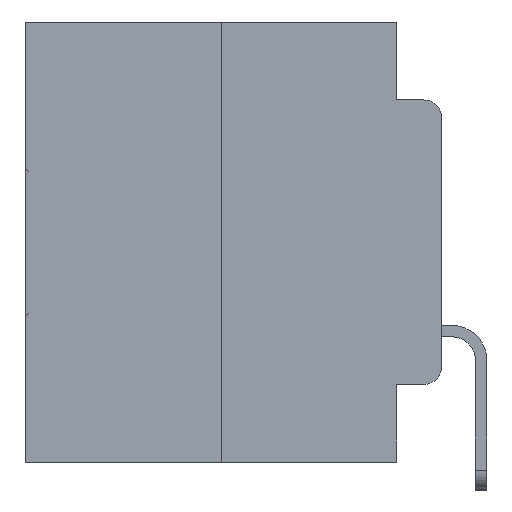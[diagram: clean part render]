
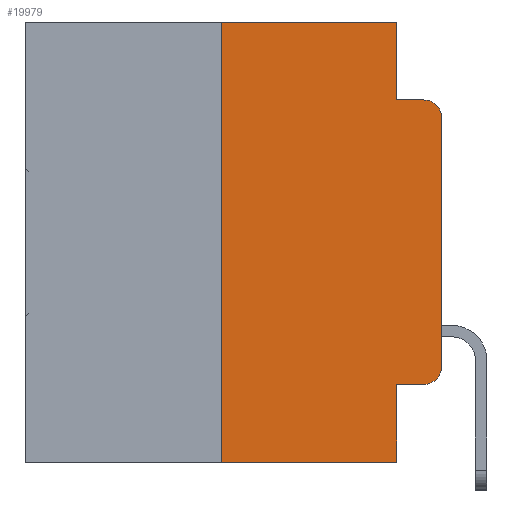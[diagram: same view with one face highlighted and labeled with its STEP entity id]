
A CAD part, left-side view. The second image highlights one B-rep face of the part: STEP entity #19979.
In plain terms, the highlighted planar face has unit normal (-1, 0, 0).
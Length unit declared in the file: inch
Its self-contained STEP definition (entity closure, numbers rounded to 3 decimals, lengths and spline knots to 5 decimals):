
#243 = ORIENTED_EDGE ( 'NONE', *, *, #19623, .F. ) ;
#289 = CARTESIAN_POINT ( 'NONE',  ( 0., 0.02, -0.0885 ) ) ;
#1287 = VECTOR ( 'NONE', #19741, 39.37008 ) ;
#1308 = LINE ( 'NONE', #17539, #7800 ) ;
#1416 = VERTEX_POINT ( 'NONE', #9421 ) ;
#2007 = EDGE_CURVE ( 'NONE', #29430, #29545, #8652, .T. ) ;
#2141 = ORIENTED_EDGE ( 'NONE', *, *, #22216, .F. ) ;
#2226 = VERTEX_POINT ( 'NONE', #16152 ) ;
#2608 = AXIS2_PLACEMENT_3D ( 'NONE', #10638, #24581, #8206 ) ;
#3212 = DIRECTION ( 'NONE',  ( 0., 0., 1. ) ) ;
#3715 = EDGE_CURVE ( 'NONE', #11096, #2226, #7783, .T. ) ;
#3716 = EDGE_LOOP ( 'NONE', ( #5643, #10127, #17434, #243, #2141, #10938, #17125, #20811, #22616, #24074 ) ) ;
#4647 = CARTESIAN_POINT ( 'NONE',  ( 0., 0.02, -0.3915 ) ) ;
#4738 = EDGE_CURVE ( 'NONE', #8073, #19058, #12789, .T. ) ;
#5018 = EDGE_CURVE ( 'NONE', #8073, #2226, #5283, .T. ) ;
#5283 = LINE ( 'NONE', #19910, #28404 ) ;
#5554 = CARTESIAN_POINT ( 'NONE',  ( 0., 0.051, -0.0885 ) ) ;
#5643 = ORIENTED_EDGE ( 'NONE', *, *, #12633, .T. ) ;
#6430 = DIRECTION ( 'NONE',  ( -1., 0., 0. ) ) ;
#7376 = EDGE_CURVE ( 'NONE', #15866, #23054, #10783, .T. ) ;
#7699 = CARTESIAN_POINT ( 'NONE',  ( 0., 0.02, -0.4115 ) ) ;
#7783 = LINE ( 'NONE', #20684, #1287 ) ;
#7800 = VECTOR ( 'NONE', #3212, 39.37008 ) ;
#7851 = DIRECTION ( 'NONE',  ( 0., -1., 0. ) ) ;
#8073 = VERTEX_POINT ( 'NONE', #18303 ) ;
#8206 = DIRECTION ( 'NONE',  ( 0., 0., -1. ) ) ;
#8372 = VECTOR ( 'NONE', #12386, 39.37008 ) ;
#8652 = CIRCLE ( 'NONE', #11125, 0.02 ) ;
#9065 = LINE ( 'NONE', #27260, #26817 ) ;
#9119 = DIRECTION ( 'NONE',  ( 0., 0., -1. ) ) ;
#9421 = CARTESIAN_POINT ( 'NONE',  ( 0., 0.051, -0.0885 ) ) ;
#10127 = ORIENTED_EDGE ( 'NONE', *, *, #7376, .T. ) ;
#10317 = CARTESIAN_POINT ( 'NONE',  ( 0., 0.473, 0. ) ) ;
#10638 = CARTESIAN_POINT ( 'NONE',  ( 0., 0.02, -0.1085 ) ) ;
#10783 = CIRCLE ( 'NONE', #2608, 0.02 ) ;
#10830 = CARTESIAN_POINT ( 'NONE',  ( 0., 0.25, 0. ) ) ;
#10938 = ORIENTED_EDGE ( 'NONE', *, *, #4738, .F. ) ;
#11086 = VECTOR ( 'NONE', #12764, 39.37008 ) ;
#11096 = VERTEX_POINT ( 'NONE', #25644 ) ;
#11125 = AXIS2_PLACEMENT_3D ( 'NONE', #4647, #6430, #18836 ) ;
#11273 = DIRECTION ( 'NONE',  ( 0., -1., 0. ) ) ;
#12113 = FACE_OUTER_BOUND ( 'NONE', #3716, .T. ) ;
#12386 = DIRECTION ( 'NONE',  ( 0., 0., -1. ) ) ;
#12442 = LINE ( 'NONE', #10317, #29729 ) ;
#12633 = EDGE_CURVE ( 'NONE', #29545, #15866, #1308, .T. ) ;
#12764 = DIRECTION ( 'NONE',  ( 0., -1., 0. ) ) ;
#12789 = LINE ( 'NONE', #29123, #24394 ) ;
#14401 = EDGE_CURVE ( 'NONE', #1416, #23054, #24208, .T. ) ;
#14715 = LINE ( 'NONE', #26202, #8372 ) ;
#15533 = DIRECTION ( 'NONE',  ( 0., -1., 0. ) ) ;
#15866 = VERTEX_POINT ( 'NONE', #20586 ) ;
#16152 = CARTESIAN_POINT ( 'NONE',  ( 0., 0.051, -0.5 ) ) ;
#16246 = PLANE ( 'NONE',  #28299 ) ;
#17125 = ORIENTED_EDGE ( 'NONE', *, *, #5018, .T. ) ;
#17434 = ORIENTED_EDGE ( 'NONE', *, *, #14401, .F. ) ;
#17539 = CARTESIAN_POINT ( 'NONE',  ( 0., 0., 0. ) ) ;
#18169 = CARTESIAN_POINT ( 'NONE',  ( 0., 0.051, 0. ) ) ;
#18303 = CARTESIAN_POINT ( 'NONE',  ( 0., 0.25, -0.5 ) ) ;
#18836 = DIRECTION ( 'NONE',  ( 0., 0., -1. ) ) ;
#19058 = VERTEX_POINT ( 'NONE', #10830 ) ;
#19623 = EDGE_CURVE ( 'NONE', #24405, #1416, #14715, .T. ) ;
#19741 = DIRECTION ( 'NONE',  ( 0., 0., -1. ) ) ;
#19778 = CARTESIAN_POINT ( 'NONE',  ( 0., 0., -0.3915 ) ) ;
#19910 = CARTESIAN_POINT ( 'NONE',  ( 0., 0.473, -0.5 ) ) ;
#19979 = ADVANCED_FACE ( 'NONE', ( #12113 ), #16246, .F. ) ;
#20586 = CARTESIAN_POINT ( 'NONE',  ( 0., 0., -0.1085 ) ) ;
#20684 = CARTESIAN_POINT ( 'NONE',  ( 0., 0.051, 0. ) ) ;
#20811 = ORIENTED_EDGE ( 'NONE', *, *, #3715, .F. ) ;
#22216 = EDGE_CURVE ( 'NONE', #19058, #24405, #12442, .T. ) ;
#22616 = ORIENTED_EDGE ( 'NONE', *, *, #25700, .T. ) ;
#23054 = VERTEX_POINT ( 'NONE', #289 ) ;
#23088 = CARTESIAN_POINT ( 'NONE',  ( 0., 0.473, 0. ) ) ;
#23191 = DIRECTION ( 'NONE',  ( 1., 0., 0. ) ) ;
#24074 = ORIENTED_EDGE ( 'NONE', *, *, #2007, .T. ) ;
#24208 = LINE ( 'NONE', #5554, #11086 ) ;
#24394 = VECTOR ( 'NONE', #28203, 39.37008 ) ;
#24405 = VERTEX_POINT ( 'NONE', #18169 ) ;
#24581 = DIRECTION ( 'NONE',  ( -1., 0., 0. ) ) ;
#25644 = CARTESIAN_POINT ( 'NONE',  ( 0., 0.051, -0.4115 ) ) ;
#25700 = EDGE_CURVE ( 'NONE', #11096, #29430, #9065, .T. ) ;
#26202 = CARTESIAN_POINT ( 'NONE',  ( 0., 0.051, 0. ) ) ;
#26817 = VECTOR ( 'NONE', #11273, 39.37008 ) ;
#27260 = CARTESIAN_POINT ( 'NONE',  ( 0., 0.051, -0.4115 ) ) ;
#28203 = DIRECTION ( 'NONE',  ( 0., 0., 1. ) ) ;
#28299 = AXIS2_PLACEMENT_3D ( 'NONE', #23088, #23191, #9119 ) ;
#28404 = VECTOR ( 'NONE', #15533, 39.37008 ) ;
#29123 = CARTESIAN_POINT ( 'NONE',  ( 0., 0.25, 0. ) ) ;
#29430 = VERTEX_POINT ( 'NONE', #7699 ) ;
#29545 = VERTEX_POINT ( 'NONE', #19778 ) ;
#29729 = VECTOR ( 'NONE', #7851, 39.37008 ) ;
